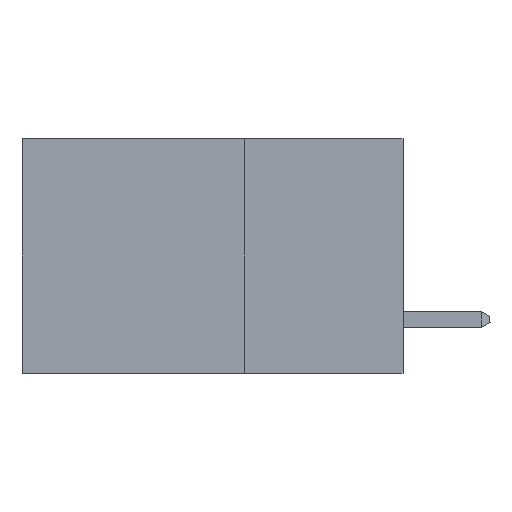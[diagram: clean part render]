
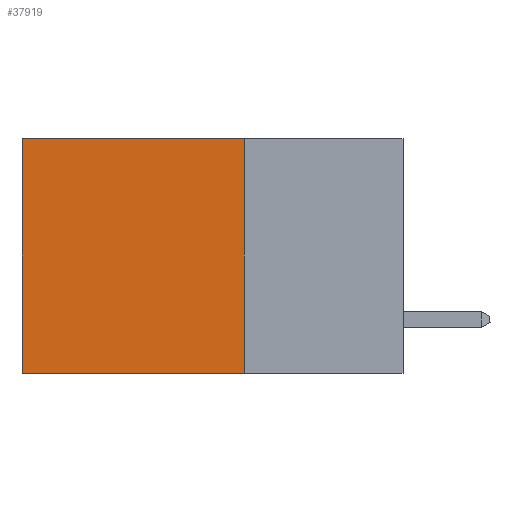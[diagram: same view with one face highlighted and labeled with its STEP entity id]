
A CAD part, left-side view. The second image highlights one B-rep face of the part: STEP entity #37919.
In plain terms, the highlighted planar face has unit normal (-1, 0, 0).
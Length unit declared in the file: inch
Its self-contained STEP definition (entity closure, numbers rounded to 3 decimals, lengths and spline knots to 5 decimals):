
#234 = ORIENTED_EDGE ( 'NONE', *, *, #18440, .T. ) ;
#1410 = EDGE_CURVE ( 'NONE', #29138, #23931, #31338, .T. ) ;
#1962 = CARTESIAN_POINT ( 'NONE',  ( 0.2875, 0.25, 0. ) ) ;
#2966 = EDGE_LOOP ( 'NONE', ( #33347, #26800, #26059, #234 ) ) ;
#3461 = LINE ( 'NONE', #38030, #14196 ) ;
#6731 = VECTOR ( 'NONE', #26949, 39.37008 ) ;
#6774 = DIRECTION ( 'NONE',  ( 1., 0., 0. ) ) ;
#7918 = DIRECTION ( 'NONE',  ( 0., 0., -1. ) ) ;
#14196 = VECTOR ( 'NONE', #16695, 39.37008 ) ;
#15640 = VECTOR ( 'NONE', #20721, 39.37008 ) ;
#16030 = CARTESIAN_POINT ( 'NONE',  ( 0.2875, 0.25, 0. ) ) ;
#16695 = DIRECTION ( 'NONE',  ( 0., 1., 0. ) ) ;
#17998 = CARTESIAN_POINT ( 'NONE',  ( 0.2875, 0.25, 0. ) ) ;
#18440 = EDGE_CURVE ( 'NONE', #21516, #29138, #36553, .T. ) ;
#19838 = CARTESIAN_POINT ( 'NONE',  ( 0.2875, 0.6, 0. ) ) ;
#20721 = DIRECTION ( 'NONE',  ( 0., 1., 0. ) ) ;
#21516 = VERTEX_POINT ( 'NONE', #17998 ) ;
#23863 = CARTESIAN_POINT ( 'NONE',  ( 0.2875, 0.6, 0. ) ) ;
#23931 = VERTEX_POINT ( 'NONE', #24033 ) ;
#24033 = CARTESIAN_POINT ( 'NONE',  ( 0.2875, 0.6, -0.37 ) ) ;
#24184 = VERTEX_POINT ( 'NONE', #26580 ) ;
#25218 = PLANE ( 'NONE',  #35156 ) ;
#25465 = DIRECTION ( 'NONE',  ( 0., 0., -1. ) ) ;
#26059 = ORIENTED_EDGE ( 'NONE', *, *, #37104, .F. ) ;
#26580 = CARTESIAN_POINT ( 'NONE',  ( 0.2875, 0.25, -0.37 ) ) ;
#26800 = ORIENTED_EDGE ( 'NONE', *, *, #31569, .F. ) ;
#26949 = DIRECTION ( 'NONE',  ( 0., 0., -1. ) ) ;
#29138 = VERTEX_POINT ( 'NONE', #19838 ) ;
#30380 = FACE_OUTER_BOUND ( 'NONE', #2966, .T. ) ;
#30403 = VECTOR ( 'NONE', #7918, 39.37008 ) ;
#31338 = LINE ( 'NONE', #23863, #30403 ) ;
#31569 = EDGE_CURVE ( 'NONE', #24184, #23931, #3461, .T. ) ;
#33016 = CARTESIAN_POINT ( 'NONE',  ( 0.2875, 0.25, 0. ) ) ;
#33347 = ORIENTED_EDGE ( 'NONE', *, *, #1410, .T. ) ;
#35156 = AXIS2_PLACEMENT_3D ( 'NONE', #16030, #6774, #25465 ) ;
#36553 = LINE ( 'NONE', #1962, #15640 ) ;
#37104 = EDGE_CURVE ( 'NONE', #21516, #24184, #39878, .T. ) ;
#37919 = ADVANCED_FACE ( 'NONE', ( #30380 ), #25218, .F. ) ;
#38030 = CARTESIAN_POINT ( 'NONE',  ( 0.2875, 0.25, -0.37 ) ) ;
#39878 = LINE ( 'NONE', #33016, #6731 ) ;
